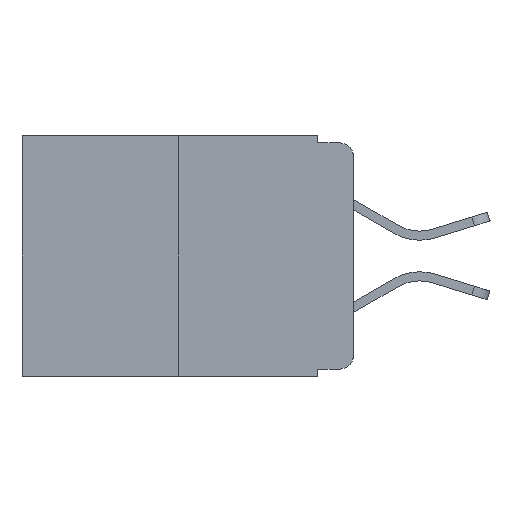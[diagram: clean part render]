
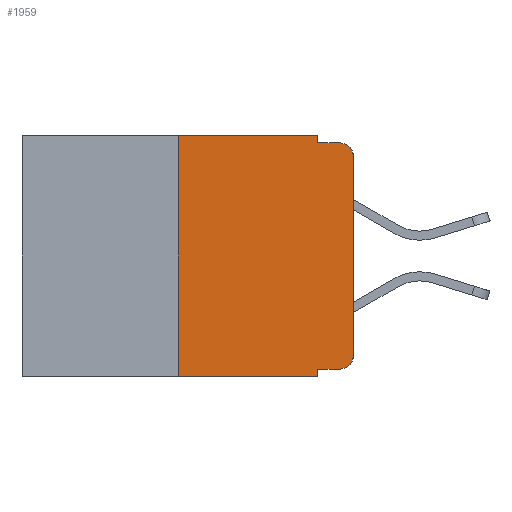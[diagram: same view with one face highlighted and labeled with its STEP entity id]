
A CAD part, left-side view. The second image highlights one B-rep face of the part: STEP entity #1959.
In plain terms, the highlighted planar face has unit normal (-1, 0, 0).
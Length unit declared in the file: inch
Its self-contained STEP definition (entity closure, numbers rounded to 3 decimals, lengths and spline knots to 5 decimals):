
#4 = EDGE_CURVE ( 'NONE', #4635, #237, #10030, .T. ) ;
#183 = ORIENTED_EDGE ( 'NONE', *, *, #9765, .T. ) ;
#237 = VERTEX_POINT ( 'NONE', #743 ) ;
#411 = ORIENTED_EDGE ( 'NONE', *, *, #10607, .F. ) ;
#467 = VERTEX_POINT ( 'NONE', #2259 ) ;
#710 = VECTOR ( 'NONE', #11383, 39.37008 ) ;
#743 = CARTESIAN_POINT ( 'NONE',  ( 0., 0.02, -0.01 ) ) ;
#756 = LINE ( 'NONE', #11838, #8598 ) ;
#925 = VECTOR ( 'NONE', #9707, 39.37008 ) ;
#956 = ORIENTED_EDGE ( 'NONE', *, *, #7340, .T. ) ;
#959 = EDGE_CURVE ( 'NONE', #8925, #10538, #12961, .T. ) ;
#1159 = EDGE_CURVE ( 'NONE', #11059, #467, #10601, .T. ) ;
#1360 = CARTESIAN_POINT ( 'NONE',  ( 0., 0.25, 0. ) ) ;
#1527 = EDGE_CURVE ( 'NONE', #10538, #9917, #3233, .T. ) ;
#1959 = ADVANCED_FACE ( 'NONE', ( #5286 ), #2924, .F. ) ;
#2259 = CARTESIAN_POINT ( 'NONE',  ( 0., 0.02, -0.333 ) ) ;
#2295 = CARTESIAN_POINT ( 'NONE',  ( 0., 0.473, 0. ) ) ;
#2428 = CARTESIAN_POINT ( 'NONE',  ( 0., 0., 0. ) ) ;
#2435 = DIRECTION ( 'NONE',  ( 0., 0., 1. ) ) ;
#2576 = ORIENTED_EDGE ( 'NONE', *, *, #1159, .T. ) ;
#2736 = CARTESIAN_POINT ( 'NONE',  ( 0., 0.25, -0.343 ) ) ;
#2924 = PLANE ( 'NONE',  #12084 ) ;
#3233 = LINE ( 'NONE', #13050, #710 ) ;
#3275 = DIRECTION ( 'NONE',  ( 0., -1., 0. ) ) ;
#3284 = VECTOR ( 'NONE', #2435, 39.37008 ) ;
#3585 = CARTESIAN_POINT ( 'NONE',  ( 0., 0.051, -0.333 ) ) ;
#3614 = VECTOR ( 'NONE', #3275, 39.37008 ) ;
#3663 = EDGE_LOOP ( 'NONE', ( #9223, #7526, #3926, #4566, #8475, #9456, #183, #411, #2576, #956 ) ) ;
#3733 = EDGE_CURVE ( 'NONE', #8463, #4635, #10466, .T. ) ;
#3748 = LINE ( 'NONE', #7733, #925 ) ;
#3926 = ORIENTED_EDGE ( 'NONE', *, *, #7014, .F. ) ;
#4152 = CARTESIAN_POINT ( 'NONE',  ( 0., 0.02, -0.03 ) ) ;
#4566 = ORIENTED_EDGE ( 'NONE', *, *, #1527, .F. ) ;
#4635 = VERTEX_POINT ( 'NONE', #9979 ) ;
#4725 = CARTESIAN_POINT ( 'NONE',  ( 0., 0.02, -0.313 ) ) ;
#4838 = CARTESIAN_POINT ( 'NONE',  ( 0., 0.051, 0. ) ) ;
#4854 = DIRECTION ( 'NONE',  ( 0., 0., -1. ) ) ;
#5268 = CARTESIAN_POINT ( 'NONE',  ( 0., 0.051, -0.333 ) ) ;
#5286 = FACE_OUTER_BOUND ( 'NONE', #3663, .T. ) ;
#5486 = DIRECTION ( 'NONE',  ( 0., 0., 1. ) ) ;
#5526 = VECTOR ( 'NONE', #6345, 39.37008 ) ;
#5755 = DIRECTION ( 'NONE',  ( 0., 0., -1. ) ) ;
#5782 = DIRECTION ( 'NONE',  ( -1., 0., 0. ) ) ;
#6003 = CARTESIAN_POINT ( 'NONE',  ( 0., 0.051, -0.01 ) ) ;
#6117 = CARTESIAN_POINT ( 'NONE',  ( 0., 0.051, -0.343 ) ) ;
#6345 = DIRECTION ( 'NONE',  ( 0., -1., 0. ) ) ;
#6846 = DIRECTION ( 'NONE',  ( 0., 0., -1. ) ) ;
#7014 = EDGE_CURVE ( 'NONE', #9917, #237, #11496, .T. ) ;
#7222 = DIRECTION ( 'NONE',  ( 0., -1., 0. ) ) ;
#7340 = EDGE_CURVE ( 'NONE', #467, #8463, #10732, .T. ) ;
#7397 = VERTEX_POINT ( 'NONE', #2736 ) ;
#7526 = ORIENTED_EDGE ( 'NONE', *, *, #4, .T. ) ;
#7733 = CARTESIAN_POINT ( 'NONE',  ( 0., 0.473, -0.343 ) ) ;
#8463 = VERTEX_POINT ( 'NONE', #10741 ) ;
#8475 = ORIENTED_EDGE ( 'NONE', *, *, #959, .F. ) ;
#8494 = VECTOR ( 'NONE', #5486, 39.37008 ) ;
#8598 = VECTOR ( 'NONE', #12766, 39.37008 ) ;
#8871 = DIRECTION ( 'NONE',  ( 1., 0., 0. ) ) ;
#8925 = VERTEX_POINT ( 'NONE', #9597 ) ;
#9223 = ORIENTED_EDGE ( 'NONE', *, *, #3733, .T. ) ;
#9258 = CARTESIAN_POINT ( 'NONE',  ( 0., 0.051, -0.01 ) ) ;
#9456 = ORIENTED_EDGE ( 'NONE', *, *, #9543, .F. ) ;
#9543 = EDGE_CURVE ( 'NONE', #7397, #8925, #11190, .T. ) ;
#9597 = CARTESIAN_POINT ( 'NONE',  ( 0., 0.25, 0. ) ) ;
#9707 = DIRECTION ( 'NONE',  ( 0., -1., 0. ) ) ;
#9765 = EDGE_CURVE ( 'NONE', #7397, #12698, #3748, .T. ) ;
#9917 = VERTEX_POINT ( 'NONE', #6003 ) ;
#9979 = CARTESIAN_POINT ( 'NONE',  ( 0., 0., -0.03 ) ) ;
#10030 = CIRCLE ( 'NONE', #10731, 0.02 ) ;
#10466 = LINE ( 'NONE', #2428, #8494 ) ;
#10538 = VERTEX_POINT ( 'NONE', #4838 ) ;
#10601 = LINE ( 'NONE', #5268, #12810 ) ;
#10607 = EDGE_CURVE ( 'NONE', #11059, #12698, #756, .T. ) ;
#10731 = AXIS2_PLACEMENT_3D ( 'NONE', #4152, #5782, #6846 ) ;
#10732 = CIRCLE ( 'NONE', #11826, 0.02 ) ;
#10741 = CARTESIAN_POINT ( 'NONE',  ( 0., 0., -0.313 ) ) ;
#10787 = CARTESIAN_POINT ( 'NONE',  ( 0., 0.473, 0. ) ) ;
#11059 = VERTEX_POINT ( 'NONE', #3585 ) ;
#11190 = LINE ( 'NONE', #1360, #3284 ) ;
#11383 = DIRECTION ( 'NONE',  ( 0., 0., -1. ) ) ;
#11496 = LINE ( 'NONE', #9258, #3614 ) ;
#11616 = DIRECTION ( 'NONE',  ( -1., 0., 0. ) ) ;
#11826 = AXIS2_PLACEMENT_3D ( 'NONE', #4725, #11616, #5755 ) ;
#11838 = CARTESIAN_POINT ( 'NONE',  ( 0., 0.051, 0. ) ) ;
#12084 = AXIS2_PLACEMENT_3D ( 'NONE', #2295, #8871, #4854 ) ;
#12698 = VERTEX_POINT ( 'NONE', #6117 ) ;
#12766 = DIRECTION ( 'NONE',  ( 0., 0., -1. ) ) ;
#12810 = VECTOR ( 'NONE', #7222, 39.37008 ) ;
#12961 = LINE ( 'NONE', #10787, #5526 ) ;
#13050 = CARTESIAN_POINT ( 'NONE',  ( 0., 0.051, 0. ) ) ;
